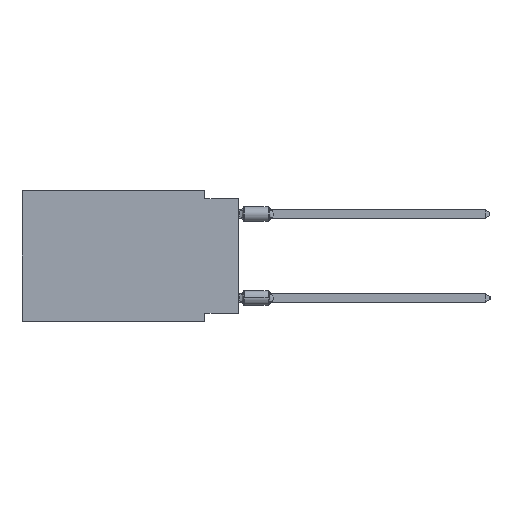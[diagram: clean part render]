
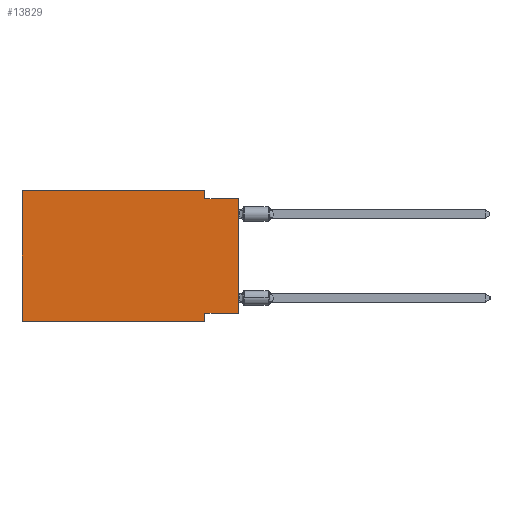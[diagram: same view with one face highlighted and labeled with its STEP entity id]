
A CAD part, left-side view. The second image highlights one B-rep face of the part: STEP entity #13829.
In plain terms, the highlighted planar face has unit normal (-1, 0, 0).
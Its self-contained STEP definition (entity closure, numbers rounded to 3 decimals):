
#10 = CARTESIAN_POINT ( 'NONE',  ( 0., 2.54, 0. ) ) ;
#165 = EDGE_CURVE ( 'NONE', #23973, #17344, #5029, .T. ) ;
#203 = FACE_OUTER_BOUND ( 'NONE', #3943, .T. ) ;
#353 = ORIENTED_EDGE ( 'NONE', *, *, #30974, .F. ) ;
#1504 = DIRECTION ( 'NONE',  ( 0., 0., 1. ) ) ;
#2002 = VECTOR ( 'NONE', #9509, 1000. ) ;
#2668 = VERTEX_POINT ( 'NONE', #12675 ) ;
#3692 = EDGE_CURVE ( 'NONE', #16024, #23973, #17778, .T. ) ;
#3943 = EDGE_LOOP ( 'NONE', ( #7340, #25871, #5208, #19312, #353, #34106, #8157, #15302 ) ) ;
#5029 = LINE ( 'NONE', #10, #6341 ) ;
#5208 = ORIENTED_EDGE ( 'NONE', *, *, #165, .F. ) ;
#6341 = VECTOR ( 'NONE', #35283, 1000. ) ;
#6570 = CARTESIAN_POINT ( 'NONE',  ( 0., 16.383, 0. ) ) ;
#6773 = EDGE_CURVE ( 'NONE', #17344, #18935, #9199, .T. ) ;
#7340 = ORIENTED_EDGE ( 'NONE', *, *, #7518, .T. ) ;
#7518 = EDGE_CURVE ( 'NONE', #34406, #18935, #9021, .T. ) ;
#7656 = CARTESIAN_POINT ( 'NONE',  ( 0., 2.54, 0. ) ) ;
#8157 = ORIENTED_EDGE ( 'NONE', *, *, #32945, .F. ) ;
#9021 = LINE ( 'NONE', #28712, #31224 ) ;
#9199 = LINE ( 'NONE', #25692, #28894 ) ;
#9509 = DIRECTION ( 'NONE',  ( 0., 1., 0. ) ) ;
#10701 = LINE ( 'NONE', #17105, #26700 ) ;
#10833 = CARTESIAN_POINT ( 'NONE',  ( 0., 0., -9.271 ) ) ;
#11419 = EDGE_CURVE ( 'NONE', #34406, #2668, #20415, .T. ) ;
#12033 = VECTOR ( 'NONE', #31221, 1000. ) ;
#12675 = CARTESIAN_POINT ( 'NONE',  ( 0., 2.54, -9.271 ) ) ;
#13596 = CARTESIAN_POINT ( 'NONE',  ( 0., 2.54, -0.635 ) ) ;
#13651 = CARTESIAN_POINT ( 'NONE',  ( 0., 16.383, -9.906 ) ) ;
#13829 = ADVANCED_FACE ( 'NONE', ( #203 ), #21663, .F. ) ;
#13971 = DIRECTION ( 'NONE',  ( 0., 0., -1. ) ) ;
#15302 = ORIENTED_EDGE ( 'NONE', *, *, #11419, .F. ) ;
#16024 = VERTEX_POINT ( 'NONE', #31859 ) ;
#17105 = CARTESIAN_POINT ( 'NONE',  ( 0., 2.54, -9.906 ) ) ;
#17344 = VERTEX_POINT ( 'NONE', #13596 ) ;
#17481 = DIRECTION ( 'NONE',  ( 0., 0., 1. ) ) ;
#17778 = LINE ( 'NONE', #33542, #12033 ) ;
#18527 = DIRECTION ( 'NONE',  ( 0., -1., 0. ) ) ;
#18638 = DIRECTION ( 'NONE',  ( 1., 0., 0. ) ) ;
#18935 = VERTEX_POINT ( 'NONE', #27858 ) ;
#19267 = DIRECTION ( 'NONE',  ( 0., 0., -1. ) ) ;
#19312 = ORIENTED_EDGE ( 'NONE', *, *, #3692, .F. ) ;
#20415 = LINE ( 'NONE', #28304, #2002 ) ;
#21663 = PLANE ( 'NONE',  #22610 ) ;
#22610 = AXIS2_PLACEMENT_3D ( 'NONE', #27409, #18638, #13971 ) ;
#23973 = VERTEX_POINT ( 'NONE', #7656 ) ;
#24889 = VECTOR ( 'NONE', #17481, 1000. ) ;
#25692 = CARTESIAN_POINT ( 'NONE',  ( 0., 0., -0.635 ) ) ;
#25871 = ORIENTED_EDGE ( 'NONE', *, *, #6773, .F. ) ;
#26262 = LINE ( 'NONE', #6570, #24889 ) ;
#26700 = VECTOR ( 'NONE', #19267, 1000. ) ;
#26780 = CARTESIAN_POINT ( 'NONE',  ( 0., 16.383, -9.906 ) ) ;
#26989 = EDGE_CURVE ( 'NONE', #27326, #31825, #32150, .T. ) ;
#27326 = VERTEX_POINT ( 'NONE', #13651 ) ;
#27409 = CARTESIAN_POINT ( 'NONE',  ( 0., 16.383, 0. ) ) ;
#27858 = CARTESIAN_POINT ( 'NONE',  ( 0., 0., -0.635 ) ) ;
#28304 = CARTESIAN_POINT ( 'NONE',  ( 0., 0., -9.271 ) ) ;
#28712 = CARTESIAN_POINT ( 'NONE',  ( 0., 0., 0. ) ) ;
#28894 = VECTOR ( 'NONE', #31401, 1000. ) ;
#30974 = EDGE_CURVE ( 'NONE', #27326, #16024, #26262, .T. ) ;
#31221 = DIRECTION ( 'NONE',  ( 0., -1., 0. ) ) ;
#31224 = VECTOR ( 'NONE', #1504, 1000. ) ;
#31401 = DIRECTION ( 'NONE',  ( 0., -1., 0. ) ) ;
#31825 = VERTEX_POINT ( 'NONE', #34777 ) ;
#31859 = CARTESIAN_POINT ( 'NONE',  ( 0., 16.383, 0. ) ) ;
#32006 = VECTOR ( 'NONE', #18527, 1000. ) ;
#32150 = LINE ( 'NONE', #26780, #32006 ) ;
#32945 = EDGE_CURVE ( 'NONE', #2668, #31825, #10701, .T. ) ;
#33542 = CARTESIAN_POINT ( 'NONE',  ( 0., 16.383, 0. ) ) ;
#34106 = ORIENTED_EDGE ( 'NONE', *, *, #26989, .T. ) ;
#34406 = VERTEX_POINT ( 'NONE', #10833 ) ;
#34777 = CARTESIAN_POINT ( 'NONE',  ( 0., 2.54, -9.906 ) ) ;
#35283 = DIRECTION ( 'NONE',  ( 0., 0., -1. ) ) ;
